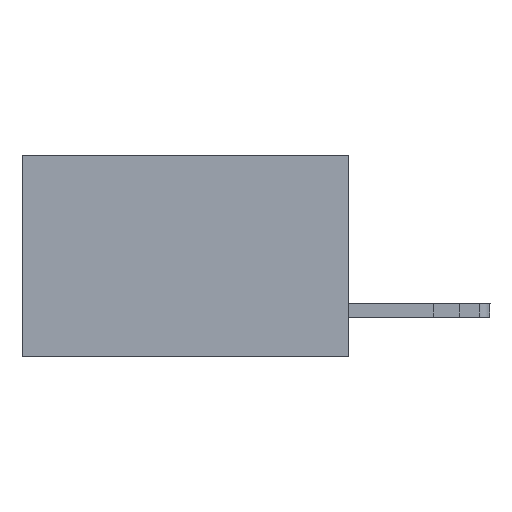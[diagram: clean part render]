
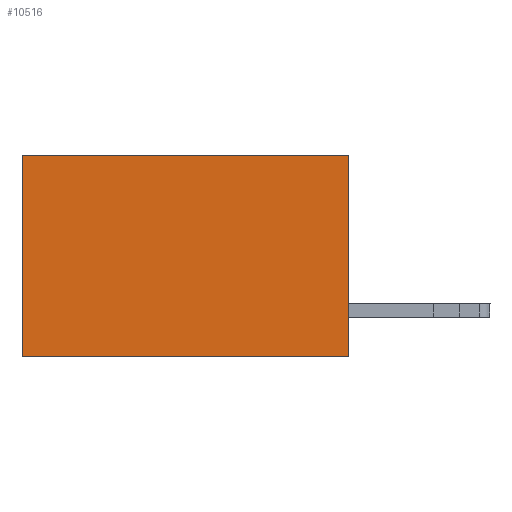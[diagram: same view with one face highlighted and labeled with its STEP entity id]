
A CAD part, left-side view. The second image highlights one B-rep face of the part: STEP entity #10516.
In plain terms, the highlighted planar face has unit normal (-1, 0, 0).
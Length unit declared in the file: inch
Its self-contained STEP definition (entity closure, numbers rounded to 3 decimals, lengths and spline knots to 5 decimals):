
#576 = DIRECTION ( 'NONE',  ( 0., 0., -1. ) ) ;
#611 = EDGE_CURVE ( 'NONE', #1634, #21553, #5452, .T. ) ;
#728 = VECTOR ( 'NONE', #7930, 39.37008 ) ;
#806 = CARTESIAN_POINT ( 'NONE',  ( 0.298, 0., 0. ) ) ;
#910 = LINE ( 'NONE', #806, #18869 ) ;
#1484 = VECTOR ( 'NONE', #576, 39.37008 ) ;
#1634 = VERTEX_POINT ( 'NONE', #10941 ) ;
#1851 = AXIS2_PLACEMENT_3D ( 'NONE', #21482, #6475, #17987 ) ;
#2676 = DIRECTION ( 'NONE',  ( 0., 0., -1. ) ) ;
#3590 = EDGE_CURVE ( 'NONE', #21553, #19828, #18782, .T. ) ;
#5132 = CARTESIAN_POINT ( 'NONE',  ( 0.298, 0., -0.37 ) ) ;
#5452 = LINE ( 'NONE', #18797, #16158 ) ;
#6475 = DIRECTION ( 'NONE',  ( 1., 0., 0. ) ) ;
#6542 = EDGE_CURVE ( 'NONE', #13348, #19828, #10794, .T. ) ;
#7078 = CARTESIAN_POINT ( 'NONE',  ( 0.298, 0.6, 0. ) ) ;
#7813 = ORIENTED_EDGE ( 'NONE', *, *, #6542, .F. ) ;
#7901 = CARTESIAN_POINT ( 'NONE',  ( 0.298, 0.6, -0.37 ) ) ;
#7930 = DIRECTION ( 'NONE',  ( 0., 1., 0. ) ) ;
#10516 = ADVANCED_FACE ( 'NONE', ( #16127 ), #14802, .F. ) ;
#10794 = LINE ( 'NONE', #10907, #728 ) ;
#10907 = CARTESIAN_POINT ( 'NONE',  ( 0.298, 0., -0.37 ) ) ;
#10941 = CARTESIAN_POINT ( 'NONE',  ( 0.298, 0., 0. ) ) ;
#13348 = VERTEX_POINT ( 'NONE', #5132 ) ;
#14063 = ORIENTED_EDGE ( 'NONE', *, *, #16287, .F. ) ;
#14802 = PLANE ( 'NONE',  #1851 ) ;
#15487 = ORIENTED_EDGE ( 'NONE', *, *, #3590, .T. ) ;
#16127 = FACE_OUTER_BOUND ( 'NONE', #16847, .T. ) ;
#16158 = VECTOR ( 'NONE', #18911, 39.37008 ) ;
#16287 = EDGE_CURVE ( 'NONE', #1634, #13348, #910, .T. ) ;
#16667 = ORIENTED_EDGE ( 'NONE', *, *, #611, .T. ) ;
#16847 = EDGE_LOOP ( 'NONE', ( #15487, #7813, #14063, #16667 ) ) ;
#17987 = DIRECTION ( 'NONE',  ( 0., 0., -1. ) ) ;
#18782 = LINE ( 'NONE', #7078, #1484 ) ;
#18797 = CARTESIAN_POINT ( 'NONE',  ( 0.298, 0., 0. ) ) ;
#18869 = VECTOR ( 'NONE', #2676, 39.37008 ) ;
#18911 = DIRECTION ( 'NONE',  ( 0., 1., 0. ) ) ;
#19058 = CARTESIAN_POINT ( 'NONE',  ( 0.298, 0.6, 0. ) ) ;
#19828 = VERTEX_POINT ( 'NONE', #7901 ) ;
#21482 = CARTESIAN_POINT ( 'NONE',  ( 0.298, 0., 0. ) ) ;
#21553 = VERTEX_POINT ( 'NONE', #19058 ) ;
